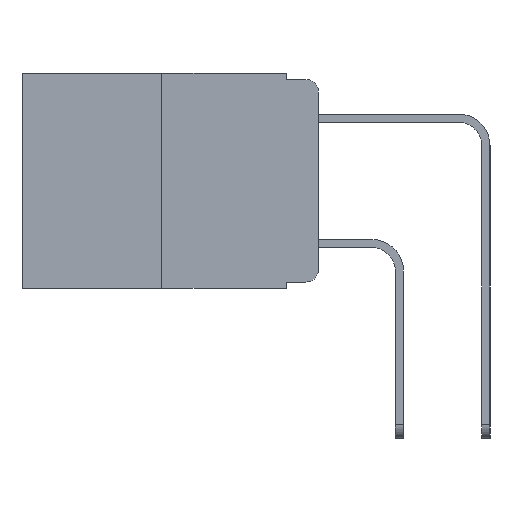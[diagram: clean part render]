
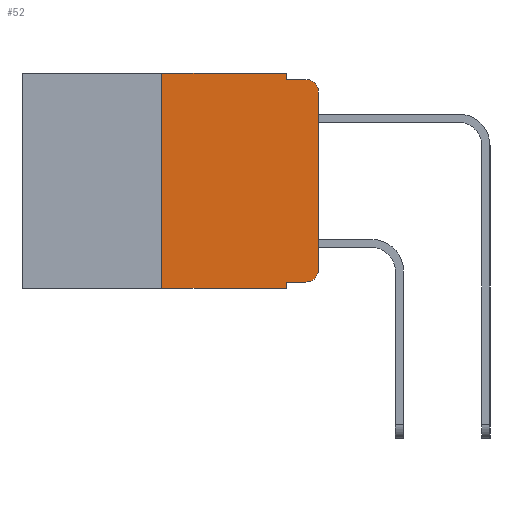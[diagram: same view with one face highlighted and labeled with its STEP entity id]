
A CAD part, left-side view. The second image highlights one B-rep face of the part: STEP entity #52.
In plain terms, the highlighted planar face has unit normal (-1, 0, 0).
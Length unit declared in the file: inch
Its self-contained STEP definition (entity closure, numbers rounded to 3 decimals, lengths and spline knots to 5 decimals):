
#52 = ADVANCED_FACE ( 'NONE', ( #2169 ), #5801, .F. ) ;
#356 = EDGE_CURVE ( 'NONE', #10290, #6616, #1130, .T. ) ;
#1130 = LINE ( 'NONE', #2849, #4407 ) ;
#1228 = EDGE_CURVE ( 'NONE', #6616, #4909, #8533, .T. ) ;
#1366 = ORIENTED_EDGE ( 'NONE', *, *, #2103, .T. ) ;
#1379 = LINE ( 'NONE', #2379, #13277 ) ;
#1637 = VECTOR ( 'NONE', #8405, 39.37008 ) ;
#1744 = ORIENTED_EDGE ( 'NONE', *, *, #3823, .F. ) ;
#1792 = ORIENTED_EDGE ( 'NONE', *, *, #356, .F. ) ;
#2067 = ORIENTED_EDGE ( 'NONE', *, *, #1228, .F. ) ;
#2103 = EDGE_CURVE ( 'NONE', #12200, #4909, #9984, .T. ) ;
#2169 = FACE_OUTER_BOUND ( 'NONE', #6996, .T. ) ;
#2379 = CARTESIAN_POINT ( 'NONE',  ( 0., 0.25, 0. ) ) ;
#2491 = DIRECTION ( 'NONE',  ( 0., -1., 0. ) ) ;
#2502 = CARTESIAN_POINT ( 'NONE',  ( 0., 0.02, -0.01 ) ) ;
#2505 = DIRECTION ( 'NONE',  ( -1., 0., 0. ) ) ;
#2558 = CARTESIAN_POINT ( 'NONE',  ( 0., 0.02, -0.333 ) ) ;
#2849 = CARTESIAN_POINT ( 'NONE',  ( 0., 0.051, 0. ) ) ;
#2860 = CARTESIAN_POINT ( 'NONE',  ( 0., 0., 0. ) ) ;
#2904 = EDGE_CURVE ( 'NONE', #12188, #12200, #11571, .T. ) ;
#2907 = AXIS2_PLACEMENT_3D ( 'NONE', #5695, #5260, #8291 ) ;
#3380 = AXIS2_PLACEMENT_3D ( 'NONE', #6951, #15006, #8146 ) ;
#3455 = ORIENTED_EDGE ( 'NONE', *, *, #14972, .F. ) ;
#3513 = ORIENTED_EDGE ( 'NONE', *, *, #11955, .T. ) ;
#3523 = ORIENTED_EDGE ( 'NONE', *, *, #11407, .T. ) ;
#3566 = DIRECTION ( 'NONE',  ( 0., 0., -1. ) ) ;
#3823 = EDGE_CURVE ( 'NONE', #7562, #10290, #14178, .T. ) ;
#4064 = DIRECTION ( 'NONE',  ( 0., 0., 1. ) ) ;
#4407 = VECTOR ( 'NONE', #7221, 39.37008 ) ;
#4909 = VERTEX_POINT ( 'NONE', #2502 ) ;
#4933 = VECTOR ( 'NONE', #6504, 39.37008 ) ;
#5260 = DIRECTION ( 'NONE',  ( 1., 0., 0. ) ) ;
#5340 = CARTESIAN_POINT ( 'NONE',  ( 0., 0.051, -0.333 ) ) ;
#5601 = CIRCLE ( 'NONE', #3380, 0.02 ) ;
#5613 = VECTOR ( 'NONE', #3566, 39.37008 ) ;
#5695 = CARTESIAN_POINT ( 'NONE',  ( 0., 0.473, 0. ) ) ;
#5801 = PLANE ( 'NONE',  #2907 ) ;
#5949 = CARTESIAN_POINT ( 'NONE',  ( 0., 0.473, 0. ) ) ;
#6499 = VECTOR ( 'NONE', #9699, 39.37008 ) ;
#6504 = DIRECTION ( 'NONE',  ( 0., -1., 0. ) ) ;
#6616 = VERTEX_POINT ( 'NONE', #13064 ) ;
#6773 = CARTESIAN_POINT ( 'NONE',  ( 0., 0.25, 0. ) ) ;
#6951 = CARTESIAN_POINT ( 'NONE',  ( 0., 0.02, -0.313 ) ) ;
#6996 = EDGE_LOOP ( 'NONE', ( #13697, #1366, #2067, #1792, #1744, #3455, #3523, #7743, #3513, #10271 ) ) ;
#7137 = CARTESIAN_POINT ( 'NONE',  ( 0., 0.25, -0.343 ) ) ;
#7221 = DIRECTION ( 'NONE',  ( 0., 0., -1. ) ) ;
#7562 = VERTEX_POINT ( 'NONE', #6773 ) ;
#7743 = ORIENTED_EDGE ( 'NONE', *, *, #14223, .F. ) ;
#7930 = CARTESIAN_POINT ( 'NONE',  ( 0., 0.051, -0.343 ) ) ;
#8142 = LINE ( 'NONE', #5340, #4933 ) ;
#8146 = DIRECTION ( 'NONE',  ( 0., 0., -1. ) ) ;
#8291 = DIRECTION ( 'NONE',  ( 0., 0., -1. ) ) ;
#8405 = DIRECTION ( 'NONE',  ( 0., -1., 0. ) ) ;
#8442 = VECTOR ( 'NONE', #4064, 39.37008 ) ;
#8533 = LINE ( 'NONE', #14054, #6499 ) ;
#8570 = VECTOR ( 'NONE', #2491, 39.37008 ) ;
#9522 = LINE ( 'NONE', #13040, #5613 ) ;
#9561 = DIRECTION ( 'NONE',  ( 0., 0., 1. ) ) ;
#9692 = CARTESIAN_POINT ( 'NONE',  ( 0., 0.02, -0.03 ) ) ;
#9699 = DIRECTION ( 'NONE',  ( 0., -1., 0. ) ) ;
#9984 = CIRCLE ( 'NONE', #13316, 0.02 ) ;
#10271 = ORIENTED_EDGE ( 'NONE', *, *, #11205, .T. ) ;
#10290 = VERTEX_POINT ( 'NONE', #14588 ) ;
#10525 = CARTESIAN_POINT ( 'NONE',  ( 0., 0., -0.313 ) ) ;
#10857 = DIRECTION ( 'NONE',  ( 0., 0., -1. ) ) ;
#11205 = EDGE_CURVE ( 'NONE', #13236, #12188, #5601, .T. ) ;
#11407 = EDGE_CURVE ( 'NONE', #14920, #13518, #11699, .T. ) ;
#11571 = LINE ( 'NONE', #2860, #8442 ) ;
#11699 = LINE ( 'NONE', #13101, #8570 ) ;
#11955 = EDGE_CURVE ( 'NONE', #12335, #13236, #8142, .T. ) ;
#12188 = VERTEX_POINT ( 'NONE', #10525 ) ;
#12200 = VERTEX_POINT ( 'NONE', #13965 ) ;
#12335 = VERTEX_POINT ( 'NONE', #14147 ) ;
#13040 = CARTESIAN_POINT ( 'NONE',  ( 0., 0.051, 0. ) ) ;
#13064 = CARTESIAN_POINT ( 'NONE',  ( 0., 0.051, -0.01 ) ) ;
#13101 = CARTESIAN_POINT ( 'NONE',  ( 0., 0.473, -0.343 ) ) ;
#13236 = VERTEX_POINT ( 'NONE', #2558 ) ;
#13277 = VECTOR ( 'NONE', #9561, 39.37008 ) ;
#13316 = AXIS2_PLACEMENT_3D ( 'NONE', #9692, #2505, #10857 ) ;
#13518 = VERTEX_POINT ( 'NONE', #7930 ) ;
#13697 = ORIENTED_EDGE ( 'NONE', *, *, #2904, .T. ) ;
#13965 = CARTESIAN_POINT ( 'NONE',  ( 0., 0., -0.03 ) ) ;
#14054 = CARTESIAN_POINT ( 'NONE',  ( 0., 0.051, -0.01 ) ) ;
#14147 = CARTESIAN_POINT ( 'NONE',  ( 0., 0.051, -0.333 ) ) ;
#14178 = LINE ( 'NONE', #5949, #1637 ) ;
#14223 = EDGE_CURVE ( 'NONE', #12335, #13518, #9522, .T. ) ;
#14588 = CARTESIAN_POINT ( 'NONE',  ( 0., 0.051, 0. ) ) ;
#14920 = VERTEX_POINT ( 'NONE', #7137 ) ;
#14972 = EDGE_CURVE ( 'NONE', #14920, #7562, #1379, .T. ) ;
#15006 = DIRECTION ( 'NONE',  ( -1., 0., 0. ) ) ;
